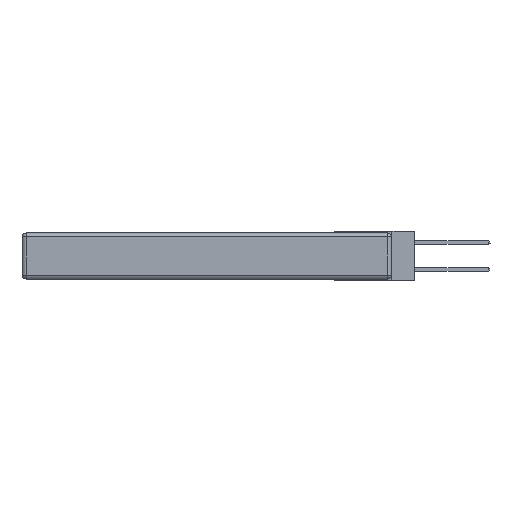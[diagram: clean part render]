
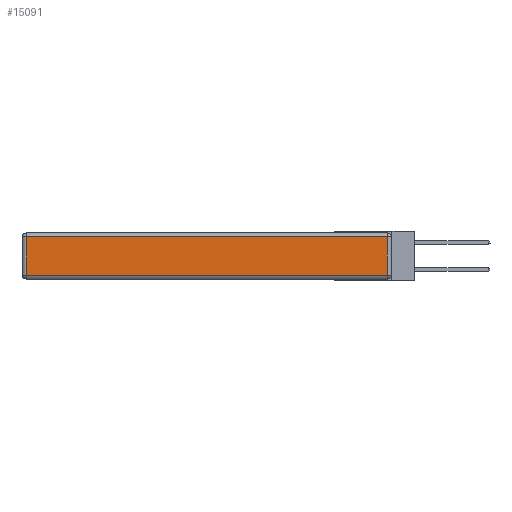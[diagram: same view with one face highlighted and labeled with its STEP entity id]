
A CAD part, left-side view. The second image highlights one B-rep face of the part: STEP entity #15091.
In plain terms, the highlighted planar face has unit normal (-1, 0, 0).
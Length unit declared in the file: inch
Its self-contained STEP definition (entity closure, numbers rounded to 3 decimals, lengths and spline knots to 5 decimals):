
#450 = ORIENTED_EDGE ( 'NONE', *, *, #563, .T. ) ;
#532 = CARTESIAN_POINT ( 'NONE',  ( 0., 2.75, -0.03 ) ) ;
#563 = EDGE_CURVE ( 'NONE', #9585, #15746, #4011, .T. ) ;
#861 = DIRECTION ( 'NONE',  ( 0., -1., 0. ) ) ;
#2242 = DIRECTION ( 'NONE',  ( 0., 0., -1. ) ) ;
#2624 = VECTOR ( 'NONE', #8640, 39.37008 ) ;
#2675 = CARTESIAN_POINT ( 'NONE',  ( 0., 0.03, -0.313 ) ) ;
#3126 = CARTESIAN_POINT ( 'NONE',  ( 0., 0.03, -0.343 ) ) ;
#4011 = LINE ( 'NONE', #14985, #4523 ) ;
#4523 = VECTOR ( 'NONE', #2242, 39.37008 ) ;
#6153 = LINE ( 'NONE', #10295, #16104 ) ;
#8640 = DIRECTION ( 'NONE',  ( 0., 1., 0. ) ) ;
#8717 = EDGE_CURVE ( 'NONE', #15746, #9721, #6153, .T. ) ;
#9417 = AXIS2_PLACEMENT_3D ( 'NONE', #18502, #10594, #13773 ) ;
#9585 = VERTEX_POINT ( 'NONE', #18929 ) ;
#9719 = DIRECTION ( 'NONE',  ( 0., 0., 1. ) ) ;
#9721 = VERTEX_POINT ( 'NONE', #2675 ) ;
#10295 = CARTESIAN_POINT ( 'NONE',  ( 0., 0., -0.313 ) ) ;
#10594 = DIRECTION ( 'NONE',  ( -1., 0., 0. ) ) ;
#13669 = FACE_OUTER_BOUND ( 'NONE', #15187, .T. ) ;
#13773 = DIRECTION ( 'NONE',  ( 0., 0., 1. ) ) ;
#13974 = ORIENTED_EDGE ( 'NONE', *, *, #16912, .T. ) ;
#14648 = CARTESIAN_POINT ( 'NONE',  ( 0., 2.72, -0.313 ) ) ;
#14828 = CARTESIAN_POINT ( 'NONE',  ( 0., 0.03, -0.03 ) ) ;
#14985 = CARTESIAN_POINT ( 'NONE',  ( 0., 2.72, -0.343 ) ) ;
#15082 = LINE ( 'NONE', #3126, #18104 ) ;
#15091 = ADVANCED_FACE ( 'NONE', ( #13669 ), #20317, .T. ) ;
#15187 = EDGE_LOOP ( 'NONE', ( #19915, #13974, #17866, #450 ) ) ;
#15746 = VERTEX_POINT ( 'NONE', #14648 ) ;
#16104 = VECTOR ( 'NONE', #861, 39.37008 ) ;
#16615 = EDGE_CURVE ( 'NONE', #19224, #9585, #19105, .T. ) ;
#16912 = EDGE_CURVE ( 'NONE', #9721, #19224, #15082, .T. ) ;
#17866 = ORIENTED_EDGE ( 'NONE', *, *, #16615, .T. ) ;
#18104 = VECTOR ( 'NONE', #9719, 39.37008 ) ;
#18502 = CARTESIAN_POINT ( 'NONE',  ( 0., 0., -0.343 ) ) ;
#18929 = CARTESIAN_POINT ( 'NONE',  ( 0., 2.72, -0.03 ) ) ;
#19105 = LINE ( 'NONE', #532, #2624 ) ;
#19224 = VERTEX_POINT ( 'NONE', #14828 ) ;
#19915 = ORIENTED_EDGE ( 'NONE', *, *, #8717, .T. ) ;
#20317 = PLANE ( 'NONE',  #9417 ) ;
